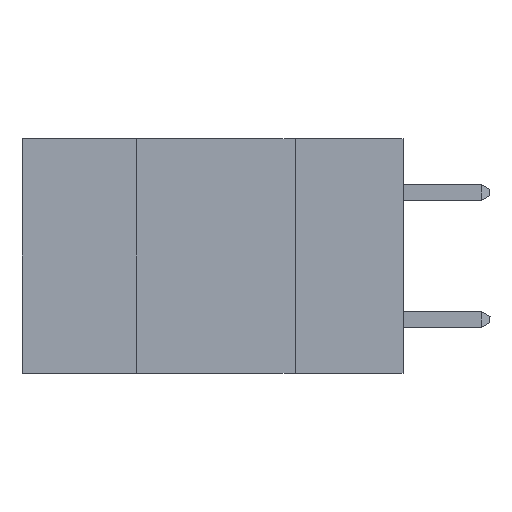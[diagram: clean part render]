
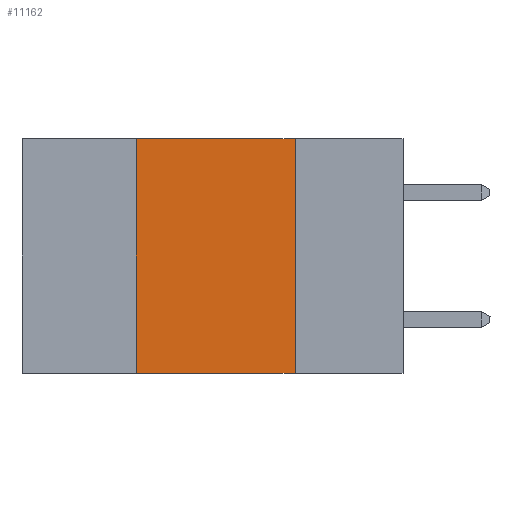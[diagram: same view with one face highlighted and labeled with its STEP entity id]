
A CAD part, left-side view. The second image highlights one B-rep face of the part: STEP entity #11162.
In plain terms, the highlighted planar face has unit normal (-1, 0, 0).
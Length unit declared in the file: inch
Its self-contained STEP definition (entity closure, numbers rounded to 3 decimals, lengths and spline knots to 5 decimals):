
#854 = CARTESIAN_POINT ( 'NONE',  ( 0., 0.42, -0.37 ) ) ;
#1113 = VECTOR ( 'NONE', #6149, 39.37008 ) ;
#1205 = EDGE_CURVE ( 'NONE', #3568, #5201, #4561, .T. ) ;
#1461 = AXIS2_PLACEMENT_3D ( 'NONE', #3142, #14218, #6479 ) ;
#1554 = EDGE_CURVE ( 'NONE', #7973, #5201, #2378, .T. ) ;
#1711 = DIRECTION ( 'NONE',  ( 0., -1., 0. ) ) ;
#1743 = VECTOR ( 'NONE', #11313, 39.37008 ) ;
#2378 = LINE ( 'NONE', #2600, #9586 ) ;
#2399 = EDGE_LOOP ( 'NONE', ( #5557, #14488, #4244, #7794 ) ) ;
#2600 = CARTESIAN_POINT ( 'NONE',  ( 0., 0.17, 0. ) ) ;
#2682 = LINE ( 'NONE', #10688, #4889 ) ;
#3142 = CARTESIAN_POINT ( 'NONE',  ( 0., 0.6, 0. ) ) ;
#3446 = CARTESIAN_POINT ( 'NONE',  ( 0., 0.6, -0.37 ) ) ;
#3568 = VERTEX_POINT ( 'NONE', #854 ) ;
#4244 = ORIENTED_EDGE ( 'NONE', *, *, #4842, .F. ) ;
#4317 = EDGE_CURVE ( 'NONE', #7732, #7973, #2682, .T. ) ;
#4561 = LINE ( 'NONE', #3446, #1743 ) ;
#4842 = EDGE_CURVE ( 'NONE', #3568, #7732, #6003, .T. ) ;
#4889 = VECTOR ( 'NONE', #1711, 39.37008 ) ;
#5201 = VERTEX_POINT ( 'NONE', #9554 ) ;
#5557 = ORIENTED_EDGE ( 'NONE', *, *, #1554, .F. ) ;
#6003 = LINE ( 'NONE', #10525, #1113 ) ;
#6149 = DIRECTION ( 'NONE',  ( 0., 0., 1. ) ) ;
#6261 = FACE_OUTER_BOUND ( 'NONE', #2399, .T. ) ;
#6479 = DIRECTION ( 'NONE',  ( 0., 0., -1. ) ) ;
#7046 = DIRECTION ( 'NONE',  ( 0., 0., -1. ) ) ;
#7732 = VERTEX_POINT ( 'NONE', #14500 ) ;
#7794 = ORIENTED_EDGE ( 'NONE', *, *, #1205, .T. ) ;
#7973 = VERTEX_POINT ( 'NONE', #12766 ) ;
#9554 = CARTESIAN_POINT ( 'NONE',  ( 0., 0.17, -0.37 ) ) ;
#9586 = VECTOR ( 'NONE', #7046, 39.37008 ) ;
#10525 = CARTESIAN_POINT ( 'NONE',  ( 0., 0.42, 0. ) ) ;
#10688 = CARTESIAN_POINT ( 'NONE',  ( 0., 0.6, 0. ) ) ;
#11162 = ADVANCED_FACE ( 'NONE', ( #6261 ), #13023, .F. ) ;
#11313 = DIRECTION ( 'NONE',  ( 0., -1., 0. ) ) ;
#12766 = CARTESIAN_POINT ( 'NONE',  ( 0., 0.17, 0. ) ) ;
#13023 = PLANE ( 'NONE',  #1461 ) ;
#14218 = DIRECTION ( 'NONE',  ( 1., 0., 0. ) ) ;
#14488 = ORIENTED_EDGE ( 'NONE', *, *, #4317, .F. ) ;
#14500 = CARTESIAN_POINT ( 'NONE',  ( 0., 0.42, 0. ) ) ;
